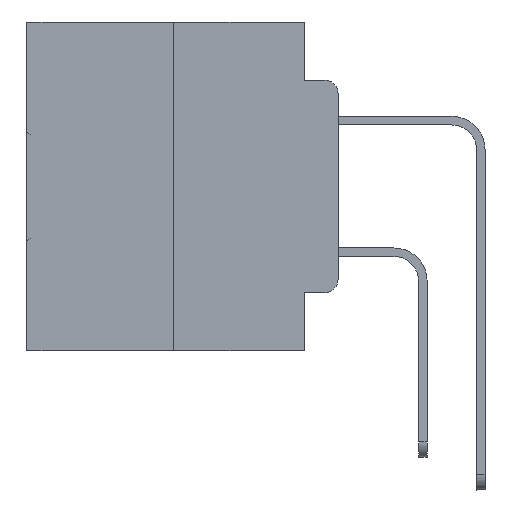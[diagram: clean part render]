
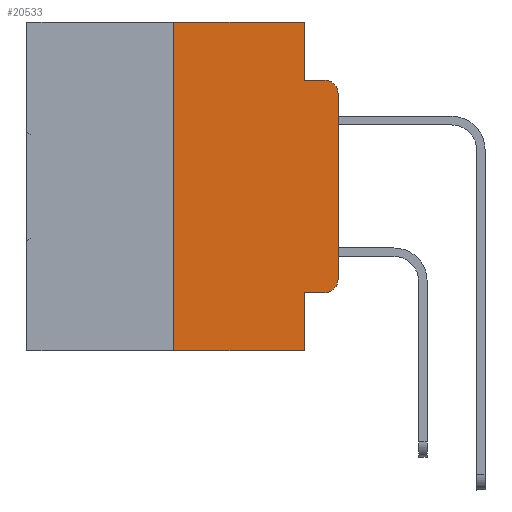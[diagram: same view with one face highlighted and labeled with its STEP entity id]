
A CAD part, left-side view. The second image highlights one B-rep face of the part: STEP entity #20533.
In plain terms, the highlighted planar face has unit normal (-1, 0, 0).
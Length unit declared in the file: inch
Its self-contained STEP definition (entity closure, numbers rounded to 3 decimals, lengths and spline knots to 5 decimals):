
#86 = VECTOR ( 'NONE', #28990, 39.37008 ) ;
#723 = VECTOR ( 'NONE', #12798, 39.37008 ) ;
#884 = ORIENTED_EDGE ( 'NONE', *, *, #15291, .F. ) ;
#1752 = DIRECTION ( 'NONE',  ( 0., 0., -1. ) ) ;
#2433 = VECTOR ( 'NONE', #26294, 39.37008 ) ;
#2753 = LINE ( 'NONE', #10021, #30009 ) ;
#2782 = PLANE ( 'NONE',  #31750 ) ;
#3277 = VERTEX_POINT ( 'NONE', #30406 ) ;
#3312 = ORIENTED_EDGE ( 'NONE', *, *, #22066, .F. ) ;
#5053 = VERTEX_POINT ( 'NONE', #11701 ) ;
#5063 = VERTEX_POINT ( 'NONE', #12027 ) ;
#5572 = CARTESIAN_POINT ( 'NONE',  ( 0., 0., -0.1085 ) ) ;
#6045 = CARTESIAN_POINT ( 'NONE',  ( 0., 0.051, -0.5 ) ) ;
#6166 = EDGE_CURVE ( 'NONE', #24463, #25206, #13472, .T. ) ;
#6176 = DIRECTION ( 'NONE',  ( 0., -1., 0. ) ) ;
#7180 = DIRECTION ( 'NONE',  ( 0., 0., 1. ) ) ;
#7356 = CARTESIAN_POINT ( 'NONE',  ( 0., 0.25, 0. ) ) ;
#7791 = EDGE_CURVE ( 'NONE', #16660, #28321, #32060, .T. ) ;
#8781 = ORIENTED_EDGE ( 'NONE', *, *, #7791, .T. ) ;
#9382 = CARTESIAN_POINT ( 'NONE',  ( 0., 0.051, 0. ) ) ;
#9433 = VECTOR ( 'NONE', #6176, 39.37008 ) ;
#10021 = CARTESIAN_POINT ( 'NONE',  ( 0., 0.051, -0.0885 ) ) ;
#10251 = AXIS2_PLACEMENT_3D ( 'NONE', #15003, #23038, #1752 ) ;
#10348 = EDGE_LOOP ( 'NONE', ( #22792, #8781, #15717, #22146, #27630, #884, #22908, #3312, #13286, #10614 ) ) ;
#10614 = ORIENTED_EDGE ( 'NONE', *, *, #33261, .T. ) ;
#10921 = VECTOR ( 'NONE', #7180, 39.37008 ) ;
#11701 = CARTESIAN_POINT ( 'NONE',  ( 0., 0.25, -0.5 ) ) ;
#11878 = EDGE_CURVE ( 'NONE', #25206, #28321, #2753, .T. ) ;
#11935 = DIRECTION ( 'NONE',  ( 0., 0., -1. ) ) ;
#12027 = CARTESIAN_POINT ( 'NONE',  ( 0., 0.051, -0.4115 ) ) ;
#12148 = LINE ( 'NONE', #33181, #10921 ) ;
#12223 = EDGE_CURVE ( 'NONE', #3277, #16660, #12148, .T. ) ;
#12798 = DIRECTION ( 'NONE',  ( 0., -1., 0. ) ) ;
#13286 = ORIENTED_EDGE ( 'NONE', *, *, #22840, .T. ) ;
#13472 = LINE ( 'NONE', #31742, #2433 ) ;
#14856 = DIRECTION ( 'NONE',  ( -1., 0., 0. ) ) ;
#15003 = CARTESIAN_POINT ( 'NONE',  ( 0., 0.02, -0.1085 ) ) ;
#15291 = EDGE_CURVE ( 'NONE', #5053, #32868, #18557, .T. ) ;
#15552 = CARTESIAN_POINT ( 'NONE',  ( 0., 0.473, -0.5 ) ) ;
#15717 = ORIENTED_EDGE ( 'NONE', *, *, #11878, .F. ) ;
#16602 = VERTEX_POINT ( 'NONE', #23568 ) ;
#16660 = VERTEX_POINT ( 'NONE', #5572 ) ;
#16695 = DIRECTION ( 'NONE',  ( 0., 0., -1. ) ) ;
#17093 = LINE ( 'NONE', #9382, #30778 ) ;
#17098 = DIRECTION ( 'NONE',  ( 0., 0., -1. ) ) ;
#17947 = CARTESIAN_POINT ( 'NONE',  ( 0., 0.473, 0. ) ) ;
#17990 = VERTEX_POINT ( 'NONE', #6045 ) ;
#18227 = CARTESIAN_POINT ( 'NONE',  ( 0., 0.25, 0. ) ) ;
#18456 = EDGE_CURVE ( 'NONE', #5053, #17990, #25647, .T. ) ;
#18557 = LINE ( 'NONE', #18227, #86 ) ;
#19662 = VECTOR ( 'NONE', #30931, 39.37008 ) ;
#20533 = ADVANCED_FACE ( 'NONE', ( #31894 ), #2782, .F. ) ;
#21480 = CIRCLE ( 'NONE', #32914, 0.02 ) ;
#21672 = DIRECTION ( 'NONE',  ( 1., 0., 0. ) ) ;
#22066 = EDGE_CURVE ( 'NONE', #5063, #17990, #17093, .T. ) ;
#22146 = ORIENTED_EDGE ( 'NONE', *, *, #6166, .F. ) ;
#22572 = CARTESIAN_POINT ( 'NONE',  ( 0., 0.02, -0.3915 ) ) ;
#22792 = ORIENTED_EDGE ( 'NONE', *, *, #12223, .T. ) ;
#22840 = EDGE_CURVE ( 'NONE', #5063, #16602, #27398, .T. ) ;
#22908 = ORIENTED_EDGE ( 'NONE', *, *, #18456, .T. ) ;
#23038 = DIRECTION ( 'NONE',  ( -1., 0., 0. ) ) ;
#23201 = DIRECTION ( 'NONE',  ( 0., -1., 0. ) ) ;
#23568 = CARTESIAN_POINT ( 'NONE',  ( 0., 0.02, -0.4115 ) ) ;
#23989 = CARTESIAN_POINT ( 'NONE',  ( 0., 0.051, -0.4115 ) ) ;
#24463 = VERTEX_POINT ( 'NONE', #32381 ) ;
#24979 = EDGE_CURVE ( 'NONE', #32868, #24463, #31406, .T. ) ;
#25206 = VERTEX_POINT ( 'NONE', #30539 ) ;
#25647 = LINE ( 'NONE', #15552, #19662 ) ;
#26294 = DIRECTION ( 'NONE',  ( 0., 0., -1. ) ) ;
#27398 = LINE ( 'NONE', #23989, #9433 ) ;
#27630 = ORIENTED_EDGE ( 'NONE', *, *, #24979, .F. ) ;
#28321 = VERTEX_POINT ( 'NONE', #32147 ) ;
#28990 = DIRECTION ( 'NONE',  ( 0., 0., 1. ) ) ;
#29687 = CARTESIAN_POINT ( 'NONE',  ( 0., 0.473, 0. ) ) ;
#30009 = VECTOR ( 'NONE', #23201, 39.37008 ) ;
#30406 = CARTESIAN_POINT ( 'NONE',  ( 0., 0., -0.3915 ) ) ;
#30539 = CARTESIAN_POINT ( 'NONE',  ( 0., 0.051, -0.0885 ) ) ;
#30778 = VECTOR ( 'NONE', #11935, 39.37008 ) ;
#30931 = DIRECTION ( 'NONE',  ( 0., -1., 0. ) ) ;
#31406 = LINE ( 'NONE', #17947, #723 ) ;
#31742 = CARTESIAN_POINT ( 'NONE',  ( 0., 0.051, 0. ) ) ;
#31750 = AXIS2_PLACEMENT_3D ( 'NONE', #29687, #21672, #16695 ) ;
#31894 = FACE_OUTER_BOUND ( 'NONE', #10348, .T. ) ;
#32060 = CIRCLE ( 'NONE', #10251, 0.02 ) ;
#32147 = CARTESIAN_POINT ( 'NONE',  ( 0., 0.02, -0.0885 ) ) ;
#32381 = CARTESIAN_POINT ( 'NONE',  ( 0., 0.051, 0. ) ) ;
#32868 = VERTEX_POINT ( 'NONE', #7356 ) ;
#32914 = AXIS2_PLACEMENT_3D ( 'NONE', #22572, #14856, #17098 ) ;
#33181 = CARTESIAN_POINT ( 'NONE',  ( 0., 0., 0. ) ) ;
#33261 = EDGE_CURVE ( 'NONE', #16602, #3277, #21480, .T. ) ;
